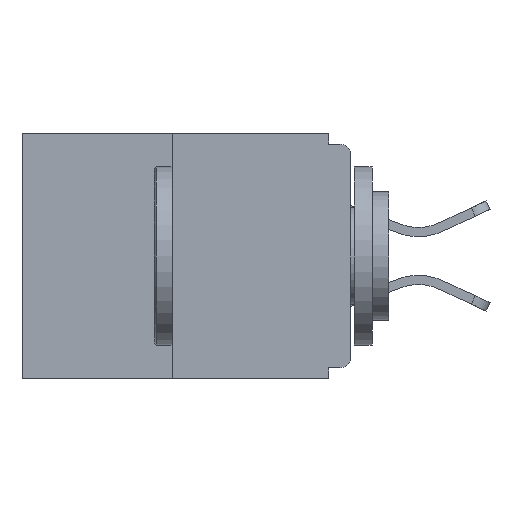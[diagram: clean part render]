
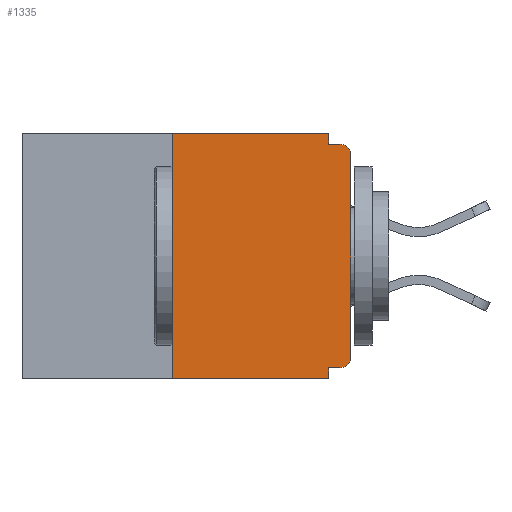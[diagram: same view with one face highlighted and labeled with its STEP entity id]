
A CAD part, left-side view. The second image highlights one B-rep face of the part: STEP entity #1335.
In plain terms, the highlighted planar face has unit normal (-1, 0, 0).
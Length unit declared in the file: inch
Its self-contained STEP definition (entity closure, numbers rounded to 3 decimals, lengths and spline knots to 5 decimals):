
#213 = VERTEX_POINT ( 'NONE', #15640 ) ;
#304 = DIRECTION ( 'NONE',  ( 0., 0., -1. ) ) ;
#880 = ORIENTED_EDGE ( 'NONE', *, *, #1351, .T. ) ;
#1046 = CARTESIAN_POINT ( 'NONE',  ( 0., 0.46, 0. ) ) ;
#1335 = ADVANCED_FACE ( 'NONE', ( #2162 ), #12763, .F. ) ;
#1351 = EDGE_CURVE ( 'NONE', #6243, #1585, #12611, .T. ) ;
#1534 = VERTEX_POINT ( 'NONE', #5754 ) ;
#1585 = VERTEX_POINT ( 'NONE', #6073 ) ;
#1636 = CARTESIAN_POINT ( 'NONE',  ( 0., 0., 0. ) ) ;
#1662 = CARTESIAN_POINT ( 'NONE',  ( 0., 0.015, -0.313 ) ) ;
#1886 = DIRECTION ( 'NONE',  ( 0., 0., -1. ) ) ;
#2162 = FACE_OUTER_BOUND ( 'NONE', #9041, .T. ) ;
#2742 = ORIENTED_EDGE ( 'NONE', *, *, #7475, .T. ) ;
#2851 = VECTOR ( 'NONE', #6779, 39.37008 ) ;
#3143 = CARTESIAN_POINT ( 'NONE',  ( 0., 0., -0.328 ) ) ;
#3169 = VERTEX_POINT ( 'NONE', #7655 ) ;
#3947 = VECTOR ( 'NONE', #1886, 39.37008 ) ;
#3955 = AXIS2_PLACEMENT_3D ( 'NONE', #15281, #7702, #10373 ) ;
#4649 = VECTOR ( 'NONE', #9231, 39.37008 ) ;
#4656 = CARTESIAN_POINT ( 'NONE',  ( 0., 0.031, -0.015 ) ) ;
#4727 = ORIENTED_EDGE ( 'NONE', *, *, #12981, .F. ) ;
#4995 = EDGE_CURVE ( 'NONE', #8916, #5861, #13655, .T. ) ;
#5628 = EDGE_CURVE ( 'NONE', #3169, #8916, #7818, .T. ) ;
#5754 = CARTESIAN_POINT ( 'NONE',  ( 0., 0.015, -0.015 ) ) ;
#5861 = VERTEX_POINT ( 'NONE', #7869 ) ;
#5995 = CIRCLE ( 'NONE', #13925, 0.015 ) ;
#6073 = CARTESIAN_POINT ( 'NONE',  ( 0., 0., -0.03 ) ) ;
#6243 = VERTEX_POINT ( 'NONE', #10113 ) ;
#6293 = ORIENTED_EDGE ( 'NONE', *, *, #15157, .T. ) ;
#6611 = LINE ( 'NONE', #3143, #4649 ) ;
#6647 = LINE ( 'NONE', #14424, #3947 ) ;
#6779 = DIRECTION ( 'NONE',  ( 0., -1., 0. ) ) ;
#6796 = EDGE_CURVE ( 'NONE', #6963, #213, #6611, .T. ) ;
#6898 = DIRECTION ( 'NONE',  ( 1., 0., 0. ) ) ;
#6963 = VERTEX_POINT ( 'NONE', #15350 ) ;
#7030 = ORIENTED_EDGE ( 'NONE', *, *, #6796, .F. ) ;
#7230 = VECTOR ( 'NONE', #12152, 39.37008 ) ;
#7475 = EDGE_CURVE ( 'NONE', #1585, #1534, #11018, .T. ) ;
#7476 = EDGE_CURVE ( 'NONE', #6963, #6243, #5995, .T. ) ;
#7655 = CARTESIAN_POINT ( 'NONE',  ( 0., 0.25, -0.343 ) ) ;
#7702 = DIRECTION ( 'NONE',  ( -1., 0., 0. ) ) ;
#7755 = CARTESIAN_POINT ( 'NONE',  ( 0., 0.031, -0.343 ) ) ;
#7805 = CARTESIAN_POINT ( 'NONE',  ( 0., 0.25, 0. ) ) ;
#7818 = LINE ( 'NONE', #14892, #14024 ) ;
#7841 = DIRECTION ( 'NONE',  ( 0., 0., 1. ) ) ;
#7869 = CARTESIAN_POINT ( 'NONE',  ( 0., 0.031, 0. ) ) ;
#8028 = DIRECTION ( 'NONE',  ( 0., -1., 0. ) ) ;
#8417 = EDGE_CURVE ( 'NONE', #13480, #1534, #11727, .T. ) ;
#8688 = ORIENTED_EDGE ( 'NONE', *, *, #4995, .F. ) ;
#8916 = VERTEX_POINT ( 'NONE', #7805 ) ;
#9041 = EDGE_LOOP ( 'NONE', ( #8688, #10923, #6293, #4727, #7030, #15504, #880, #2742, #10984, #9613 ) ) ;
#9231 = DIRECTION ( 'NONE',  ( 0., 1., 0. ) ) ;
#9296 = VECTOR ( 'NONE', #8028, 39.37008 ) ;
#9613 = ORIENTED_EDGE ( 'NONE', *, *, #9951, .F. ) ;
#9951 = EDGE_CURVE ( 'NONE', #5861, #13480, #6647, .T. ) ;
#10113 = CARTESIAN_POINT ( 'NONE',  ( 0., 0., -0.313 ) ) ;
#10172 = CARTESIAN_POINT ( 'NONE',  ( 0., 0.46, -0.343 ) ) ;
#10257 = VECTOR ( 'NONE', #7841, 39.37008 ) ;
#10355 = CARTESIAN_POINT ( 'NONE',  ( 0., 0.46, 0. ) ) ;
#10373 = DIRECTION ( 'NONE',  ( 0., 0., -1. ) ) ;
#10617 = VECTOR ( 'NONE', #13936, 39.37008 ) ;
#10923 = ORIENTED_EDGE ( 'NONE', *, *, #5628, .F. ) ;
#10984 = ORIENTED_EDGE ( 'NONE', *, *, #8417, .F. ) ;
#11003 = LINE ( 'NONE', #7755, #10617 ) ;
#11018 = CIRCLE ( 'NONE', #3955, 0.015 ) ;
#11578 = DIRECTION ( 'NONE',  ( -1., 0., 0. ) ) ;
#11727 = LINE ( 'NONE', #11740, #2851 ) ;
#11740 = CARTESIAN_POINT ( 'NONE',  ( 0., 0., -0.015 ) ) ;
#11874 = VERTEX_POINT ( 'NONE', #11969 ) ;
#11969 = CARTESIAN_POINT ( 'NONE',  ( 0., 0.031, -0.343 ) ) ;
#12152 = DIRECTION ( 'NONE',  ( 0., -1., 0. ) ) ;
#12378 = DIRECTION ( 'NONE',  ( 0., 0., 1. ) ) ;
#12611 = LINE ( 'NONE', #1636, #10257 ) ;
#12763 = PLANE ( 'NONE',  #13436 ) ;
#12928 = DIRECTION ( 'NONE',  ( 0., 0., -1. ) ) ;
#12981 = EDGE_CURVE ( 'NONE', #213, #11874, #11003, .T. ) ;
#13436 = AXIS2_PLACEMENT_3D ( 'NONE', #10355, #6898, #12928 ) ;
#13480 = VERTEX_POINT ( 'NONE', #4656 ) ;
#13655 = LINE ( 'NONE', #1046, #7230 ) ;
#13925 = AXIS2_PLACEMENT_3D ( 'NONE', #1662, #11578, #304 ) ;
#13936 = DIRECTION ( 'NONE',  ( 0., 0., -1. ) ) ;
#13974 = LINE ( 'NONE', #10172, #9296 ) ;
#14024 = VECTOR ( 'NONE', #12378, 39.37008 ) ;
#14424 = CARTESIAN_POINT ( 'NONE',  ( 0., 0.031, 0. ) ) ;
#14892 = CARTESIAN_POINT ( 'NONE',  ( 0., 0.25, 0. ) ) ;
#15157 = EDGE_CURVE ( 'NONE', #3169, #11874, #13974, .T. ) ;
#15281 = CARTESIAN_POINT ( 'NONE',  ( 0., 0.015, -0.03 ) ) ;
#15350 = CARTESIAN_POINT ( 'NONE',  ( 0., 0.015, -0.328 ) ) ;
#15504 = ORIENTED_EDGE ( 'NONE', *, *, #7476, .T. ) ;
#15640 = CARTESIAN_POINT ( 'NONE',  ( 0., 0.031, -0.328 ) ) ;
